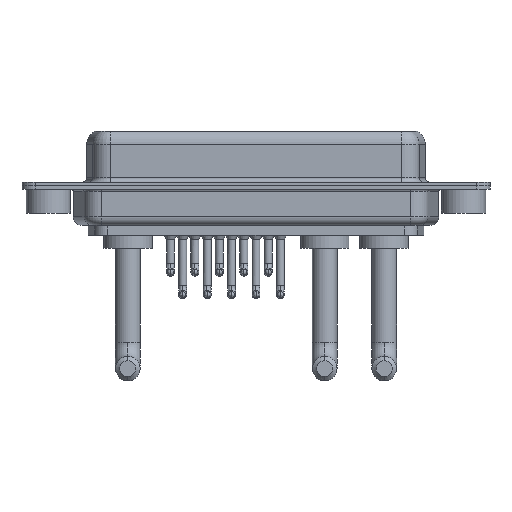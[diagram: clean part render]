
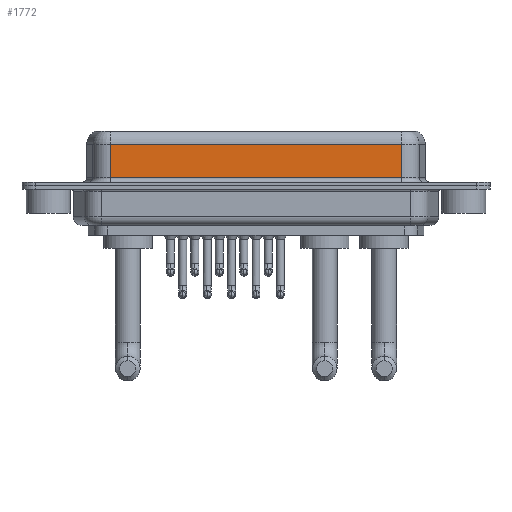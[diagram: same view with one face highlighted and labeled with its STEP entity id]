
A CAD part, front view. The second image highlights one B-rep face of the part: STEP entity #1772.
In plain terms, the highlighted planar face has unit normal (0, -1, 0).
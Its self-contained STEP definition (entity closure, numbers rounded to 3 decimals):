
#380 = DIRECTION ( 'NONE',  ( 0., 0., 1. ) ) ;
#528 = ORIENTED_EDGE ( 'NONE', *, *, #13377, .T. ) ;
#1241 = CARTESIAN_POINT ( 'NONE',  ( 40.037, -3.95, 0.9 ) ) ;
#1626 = LINE ( 'NONE', #7479, #15326 ) ;
#1772 = ADVANCED_FACE ( 'NONE', ( #2262 ), #3342, .F. ) ;
#2038 = LINE ( 'NONE', #16292, #9524 ) ;
#2262 = FACE_OUTER_BOUND ( 'NONE', #8979, .T. ) ;
#3342 = PLANE ( 'NONE',  #4946 ) ;
#4564 = DIRECTION ( 'NONE',  ( 1., 0., 0. ) ) ;
#4946 = AXIS2_PLACEMENT_3D ( 'NONE', #18337, #17972, #380 ) ;
#5604 = EDGE_CURVE ( 'NONE', #7355, #9834, #9419, .T. ) ;
#5724 = EDGE_CURVE ( 'NONE', #10134, #10811, #6925, .T. ) ;
#5729 = ORIENTED_EDGE ( 'NONE', *, *, #10647, .F. ) ;
#5995 = VECTOR ( 'NONE', #12523, 1000. ) ;
#6925 = LINE ( 'NONE', #8286, #5995 ) ;
#7224 = CARTESIAN_POINT ( 'NONE',  ( 7.013, -3.95, 0.9 ) ) ;
#7355 = VERTEX_POINT ( 'NONE', #7224 ) ;
#7479 = CARTESIAN_POINT ( 'NONE',  ( 40.037, -3.95, 6.4 ) ) ;
#8286 = CARTESIAN_POINT ( 'NONE',  ( 40.037, -3.95, 4.65 ) ) ;
#8979 = EDGE_LOOP ( 'NONE', ( #5729, #18670, #528, #15463 ) ) ;
#9419 = LINE ( 'NONE', #17755, #13985 ) ;
#9524 = VECTOR ( 'NONE', #12237, 1000. ) ;
#9834 = VERTEX_POINT ( 'NONE', #1241 ) ;
#10134 = VERTEX_POINT ( 'NONE', #13896 ) ;
#10647 = EDGE_CURVE ( 'NONE', #10134, #9834, #1626, .T. ) ;
#10811 = VERTEX_POINT ( 'NONE', #18163 ) ;
#12237 = DIRECTION ( 'NONE',  ( 0., 0., -1. ) ) ;
#12523 = DIRECTION ( 'NONE',  ( -1., 0., 0. ) ) ;
#13377 = EDGE_CURVE ( 'NONE', #10811, #7355, #2038, .T. ) ;
#13896 = CARTESIAN_POINT ( 'NONE',  ( 40.037, -3.95, 4.65 ) ) ;
#13985 = VECTOR ( 'NONE', #4564, 1000. ) ;
#15326 = VECTOR ( 'NONE', #16153, 1000. ) ;
#15463 = ORIENTED_EDGE ( 'NONE', *, *, #5604, .T. ) ;
#16153 = DIRECTION ( 'NONE',  ( 0., 0., -1. ) ) ;
#16292 = CARTESIAN_POINT ( 'NONE',  ( 7.013, -3.95, 6.4 ) ) ;
#17755 = CARTESIAN_POINT ( 'NONE',  ( 40.037, -3.95, 0.9 ) ) ;
#17972 = DIRECTION ( 'NONE',  ( 0., 1., 0. ) ) ;
#18163 = CARTESIAN_POINT ( 'NONE',  ( 7.013, -3.95, 4.65 ) ) ;
#18337 = CARTESIAN_POINT ( 'NONE',  ( 40.037, -3.95, 6.4 ) ) ;
#18670 = ORIENTED_EDGE ( 'NONE', *, *, #5724, .T. ) ;
